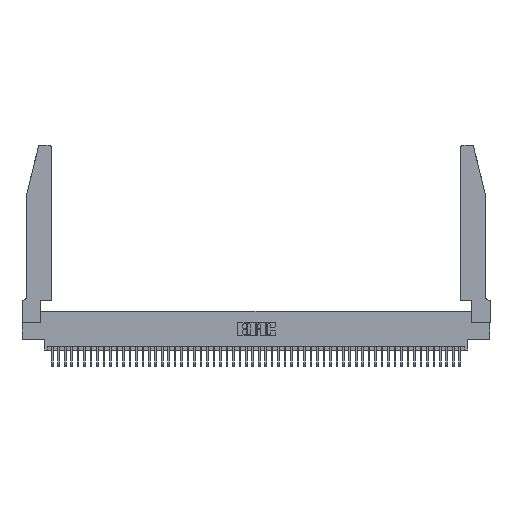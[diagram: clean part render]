
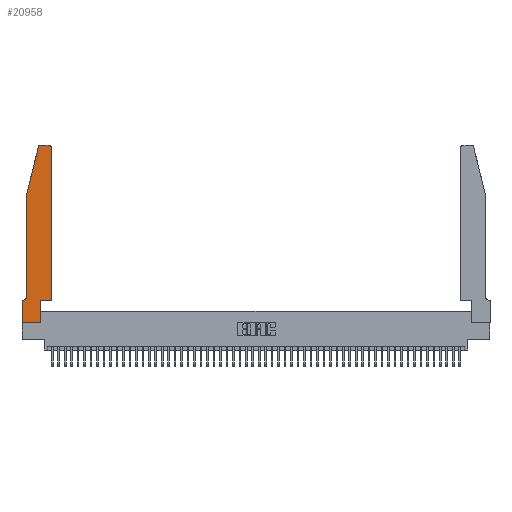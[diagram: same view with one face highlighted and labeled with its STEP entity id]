
A CAD part, top view. The second image highlights one B-rep face of the part: STEP entity #20958.
In plain terms, the highlighted planar face has unit normal (0, 0, 1).
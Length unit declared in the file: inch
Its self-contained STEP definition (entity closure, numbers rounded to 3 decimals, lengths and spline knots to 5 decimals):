
#230 = PLANE ( 'NONE',  #51909 ) ;
#305 = ORIENTED_EDGE ( 'NONE', *, *, #8812, .T. ) ;
#1030 = LINE ( 'NONE', #51768, #20941 ) ;
#1085 = CARTESIAN_POINT ( 'NONE',  ( 0.284, 2.75, 0.37 ) ) ;
#1133 = VERTEX_POINT ( 'NONE', #22326 ) ;
#1998 = ORIENTED_EDGE ( 'NONE', *, *, #2125, .T. ) ;
#2125 = EDGE_CURVE ( 'NONE', #37720, #1133, #1030, .T. ) ;
#2569 = LINE ( 'NONE', #6543, #42787 ) ;
#2683 = DIRECTION ( 'NONE',  ( 1., 0., 0. ) ) ;
#3294 = ORIENTED_EDGE ( 'NONE', *, *, #34831, .T. ) ;
#3709 = VECTOR ( 'NONE', #21880, 39.37008 ) ;
#4490 = DIRECTION ( 'NONE',  ( 1., 0., 0. ) ) ;
#5153 = VERTEX_POINT ( 'NONE', #35158 ) ;
#6034 = LINE ( 'NONE', #22074, #13214 ) ;
#6053 = DIRECTION ( 'NONE',  ( 1., 0., 0. ) ) ;
#6155 = DIRECTION ( 'NONE',  ( 0., 1., 0. ) ) ;
#6543 = CARTESIAN_POINT ( 'NONE',  ( 0., 0., 0.37 ) ) ;
#7744 = VERTEX_POINT ( 'NONE', #18455 ) ;
#8046 = CARTESIAN_POINT ( 'NONE',  ( 0.0755, 2., 0.37 ) ) ;
#8812 = EDGE_CURVE ( 'NONE', #29921, #52399, #16001, .T. ) ;
#9053 = DIRECTION ( 'NONE',  ( 0., 0., -1. ) ) ;
#10125 = AXIS2_PLACEMENT_3D ( 'NONE', #43469, #18692, #47637 ) ;
#10185 = VERTEX_POINT ( 'NONE', #46716 ) ;
#10754 = DIRECTION ( 'NONE',  ( 0., -1., 0. ) ) ;
#11203 = LINE ( 'NONE', #51680, #32001 ) ;
#11351 = ORIENTED_EDGE ( 'NONE', *, *, #27021, .T. ) ;
#13214 = VECTOR ( 'NONE', #13910, 39.37008 ) ;
#13468 = VERTEX_POINT ( 'NONE', #22913 ) ;
#13910 = DIRECTION ( 'NONE',  ( -0.239, -0.971, 0. ) ) ;
#14707 = VECTOR ( 'NONE', #42866, 39.37008 ) ;
#15249 = VECTOR ( 'NONE', #50734, 39.37008 ) ;
#16001 = LINE ( 'NONE', #17897, #14707 ) ;
#16006 = EDGE_CURVE ( 'NONE', #5153, #18480, #36882, .T. ) ;
#16145 = AXIS2_PLACEMENT_3D ( 'NONE', #33937, #9053, #38082 ) ;
#17037 = DIRECTION ( 'NONE',  ( 0., 0., 1. ) ) ;
#17614 = CARTESIAN_POINT ( 'NONE',  ( 0.4505, 0.35, 0.37 ) ) ;
#17713 = CARTESIAN_POINT ( 'NONE',  ( 0.2605, 2.75, 0.37 ) ) ;
#17897 = CARTESIAN_POINT ( 'NONE',  ( 0.0755, 0.35, 0.37 ) ) ;
#18455 = CARTESIAN_POINT ( 'NONE',  ( 0.25487, 2.72718, 0.37 ) ) ;
#18480 = VERTEX_POINT ( 'NONE', #1085 ) ;
#18692 = DIRECTION ( 'NONE',  ( 0., 0., 1. ) ) ;
#19126 = ORIENTED_EDGE ( 'NONE', *, *, #50094, .T. ) ;
#19685 = EDGE_CURVE ( 'NONE', #21840, #29921, #20425, .T. ) ;
#19733 = EDGE_LOOP ( 'NONE', ( #40402, #3294, #46715, #11351, #36341, #305, #22998, #29697, #19126, #1998, #44212, #21345 ) ) ;
#20000 = EDGE_CURVE ( 'NONE', #7744, #10185, #6034, .T. ) ;
#20425 = CIRCLE ( 'NONE', #16145, 0.07 ) ;
#20941 = VECTOR ( 'NONE', #6053, 39.37008 ) ;
#20958 = ADVANCED_FACE ( 'NONE', ( #35177 ), #230, .T. ) ;
#21345 = ORIENTED_EDGE ( 'NONE', *, *, #41612, .T. ) ;
#21840 = VERTEX_POINT ( 'NONE', #43963 ) ;
#21880 = DIRECTION ( 'NONE',  ( -1., 0., 0. ) ) ;
#22074 = CARTESIAN_POINT ( 'NONE',  ( 0.0755, 2., 0.37 ) ) ;
#22326 = CARTESIAN_POINT ( 'NONE',  ( 0.4505, 0.35, 0.37 ) ) ;
#22913 = CARTESIAN_POINT ( 'NONE',  ( 0.2865, 0., 0.37 ) ) ;
#22998 = ORIENTED_EDGE ( 'NONE', *, *, #39333, .T. ) ;
#23473 = CARTESIAN_POINT ( 'NONE',  ( 0., 0., 0.37 ) ) ;
#25243 = CARTESIAN_POINT ( 'NONE',  ( 0., 0.35, 0.37 ) ) ;
#27021 = EDGE_CURVE ( 'NONE', #10185, #21840, #46746, .T. ) ;
#29418 = DIRECTION ( 'NONE',  ( 0., 0., 1. ) ) ;
#29697 = ORIENTED_EDGE ( 'NONE', *, *, #32534, .T. ) ;
#29921 = VERTEX_POINT ( 'NONE', #39671 ) ;
#32001 = VECTOR ( 'NONE', #6155, 39.37008 ) ;
#32534 = EDGE_CURVE ( 'NONE', #47444, #13468, #34460, .T. ) ;
#33586 = CARTESIAN_POINT ( 'NONE',  ( 0., 0., 0.37 ) ) ;
#33598 = AXIS2_PLACEMENT_3D ( 'NONE', #41839, #17037, #46000 ) ;
#33937 = CARTESIAN_POINT ( 'NONE',  ( 0.0055, 0.42, 0.37 ) ) ;
#34460 = LINE ( 'NONE', #23473, #52582 ) ;
#34831 = EDGE_CURVE ( 'NONE', #18480, #7744, #40742, .T. ) ;
#35158 = CARTESIAN_POINT ( 'NONE',  ( 0.4205, 2.75, 0.37 ) ) ;
#35177 = FACE_OUTER_BOUND ( 'NONE', #19733, .T. ) ;
#35763 = VECTOR ( 'NONE', #41248, 39.37008 ) ;
#36341 = ORIENTED_EDGE ( 'NONE', *, *, #19685, .T. ) ;
#36882 = LINE ( 'NONE', #17713, #3709 ) ;
#37720 = VERTEX_POINT ( 'NONE', #52090 ) ;
#38082 = DIRECTION ( 'NONE',  ( -1., 0., 0. ) ) ;
#39333 = EDGE_CURVE ( 'NONE', #52399, #47444, #2569, .T. ) ;
#39671 = CARTESIAN_POINT ( 'NONE',  ( 0.0055, 0.35, 0.37 ) ) ;
#40402 = ORIENTED_EDGE ( 'NONE', *, *, #16006, .T. ) ;
#40742 = CIRCLE ( 'NONE', #33598, 0.03 ) ;
#41248 = DIRECTION ( 'NONE',  ( 0., -1., 0. ) ) ;
#41307 = CIRCLE ( 'NONE', #10125, 0.03 ) ;
#41612 = EDGE_CURVE ( 'NONE', #48553, #5153, #41307, .T. ) ;
#41839 = CARTESIAN_POINT ( 'NONE',  ( 0.284, 2.72, 0.37 ) ) ;
#42787 = VECTOR ( 'NONE', #10754, 39.37008 ) ;
#42866 = DIRECTION ( 'NONE',  ( -1., 0., 0. ) ) ;
#43343 = EDGE_CURVE ( 'NONE', #1133, #48553, #48281, .T. ) ;
#43469 = CARTESIAN_POINT ( 'NONE',  ( 0.4205, 2.72, 0.37 ) ) ;
#43963 = CARTESIAN_POINT ( 'NONE',  ( 0.0755, 0.42, 0.37 ) ) ;
#44212 = ORIENTED_EDGE ( 'NONE', *, *, #43343, .T. ) ;
#46000 = DIRECTION ( 'NONE',  ( 1., 0., 0. ) ) ;
#46559 = CARTESIAN_POINT ( 'NONE',  ( 0., 0.35, 0.37 ) ) ;
#46715 = ORIENTED_EDGE ( 'NONE', *, *, #20000, .T. ) ;
#46716 = CARTESIAN_POINT ( 'NONE',  ( 0.0755, 2., 0.37 ) ) ;
#46746 = LINE ( 'NONE', #8046, #35763 ) ;
#47444 = VERTEX_POINT ( 'NONE', #33586 ) ;
#47637 = DIRECTION ( 'NONE',  ( 1., 0., 0. ) ) ;
#48281 = LINE ( 'NONE', #17614, #15249 ) ;
#48553 = VERTEX_POINT ( 'NONE', #49415 ) ;
#49415 = CARTESIAN_POINT ( 'NONE',  ( 0.4505, 2.72, 0.37 ) ) ;
#50094 = EDGE_CURVE ( 'NONE', #13468, #37720, #11203, .T. ) ;
#50734 = DIRECTION ( 'NONE',  ( 0., 1., 0. ) ) ;
#51680 = CARTESIAN_POINT ( 'NONE',  ( 0.2865, 0.35, 0.37 ) ) ;
#51768 = CARTESIAN_POINT ( 'NONE',  ( 0.4505, 0.35, 0.37 ) ) ;
#51909 = AXIS2_PLACEMENT_3D ( 'NONE', #25243, #29418, #4490 ) ;
#52090 = CARTESIAN_POINT ( 'NONE',  ( 0.2865, 0.35, 0.37 ) ) ;
#52399 = VERTEX_POINT ( 'NONE', #46559 ) ;
#52582 = VECTOR ( 'NONE', #2683, 39.37008 ) ;
